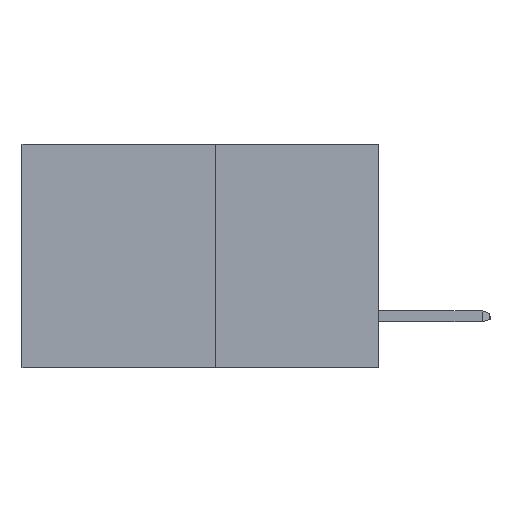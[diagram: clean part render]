
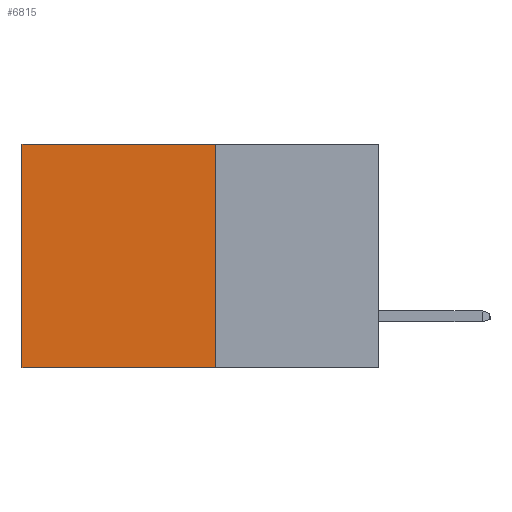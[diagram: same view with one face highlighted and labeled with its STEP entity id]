
A CAD part, left-side view. The second image highlights one B-rep face of the part: STEP entity #6815.
In plain terms, the highlighted planar face has unit normal (-1, 0, 0).
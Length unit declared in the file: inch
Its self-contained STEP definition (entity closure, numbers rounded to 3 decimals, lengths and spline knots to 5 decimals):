
#116 = VERTEX_POINT ( 'NONE', #7212 ) ;
#931 = EDGE_CURVE ( 'NONE', #116, #8930, #4935, .T. ) ;
#946 = ORIENTED_EDGE ( 'NONE', *, *, #931, .F. ) ;
#1937 = CARTESIAN_POINT ( 'NONE',  ( 0.277, 0.27, 0. ) ) ;
#2091 = EDGE_CURVE ( 'NONE', #116, #4863, #12090, .T. ) ;
#2096 = AXIS2_PLACEMENT_3D ( 'NONE', #2970, #14744, #7719 ) ;
#2970 = CARTESIAN_POINT ( 'NONE',  ( 0.277, 0.27, -0.37 ) ) ;
#3417 = CARTESIAN_POINT ( 'NONE',  ( 0.277, 0.27, -0.37 ) ) ;
#3730 = ORIENTED_EDGE ( 'NONE', *, *, #14310, .T. ) ;
#3759 = EDGE_LOOP ( 'NONE', ( #3730, #9999, #946, #4100 ) ) ;
#3875 = CARTESIAN_POINT ( 'NONE',  ( 0.277, 0.59, -0.37 ) ) ;
#4100 = ORIENTED_EDGE ( 'NONE', *, *, #2091, .T. ) ;
#4863 = VERTEX_POINT ( 'NONE', #13899 ) ;
#4935 = LINE ( 'NONE', #8735, #8446 ) ;
#5248 = LINE ( 'NONE', #3875, #11499 ) ;
#6562 = PLANE ( 'NONE',  #2096 ) ;
#6739 = VERTEX_POINT ( 'NONE', #11101 ) ;
#6815 = ADVANCED_FACE ( 'NONE', ( #11494 ), #6562, .F. ) ;
#7212 = CARTESIAN_POINT ( 'NONE',  ( 0.277, 0.27, 0. ) ) ;
#7719 = DIRECTION ( 'NONE',  ( 0., 0., -1. ) ) ;
#8446 = VECTOR ( 'NONE', #8768, 39.37008 ) ;
#8621 = VECTOR ( 'NONE', #15114, 39.37008 ) ;
#8735 = CARTESIAN_POINT ( 'NONE',  ( 0.277, 0.27, -0.37 ) ) ;
#8768 = DIRECTION ( 'NONE',  ( 0., 0., -1. ) ) ;
#8930 = VERTEX_POINT ( 'NONE', #12903 ) ;
#9999 = ORIENTED_EDGE ( 'NONE', *, *, #12808, .F. ) ;
#10058 = DIRECTION ( 'NONE',  ( 0., 1., 0. ) ) ;
#10616 = VECTOR ( 'NONE', #10058, 39.37008 ) ;
#11101 = CARTESIAN_POINT ( 'NONE',  ( 0.277, 0.59, -0.37 ) ) ;
#11363 = LINE ( 'NONE', #3417, #8621 ) ;
#11494 = FACE_OUTER_BOUND ( 'NONE', #3759, .T. ) ;
#11499 = VECTOR ( 'NONE', #12117, 39.37008 ) ;
#12090 = LINE ( 'NONE', #1937, #10616 ) ;
#12117 = DIRECTION ( 'NONE',  ( 0., 0., -1. ) ) ;
#12808 = EDGE_CURVE ( 'NONE', #8930, #6739, #11363, .T. ) ;
#12903 = CARTESIAN_POINT ( 'NONE',  ( 0.277, 0.27, -0.37 ) ) ;
#13899 = CARTESIAN_POINT ( 'NONE',  ( 0.277, 0.59, 0. ) ) ;
#14310 = EDGE_CURVE ( 'NONE', #4863, #6739, #5248, .T. ) ;
#14744 = DIRECTION ( 'NONE',  ( 1., 0., 0. ) ) ;
#15114 = DIRECTION ( 'NONE',  ( 0., 1., 0. ) ) ;
